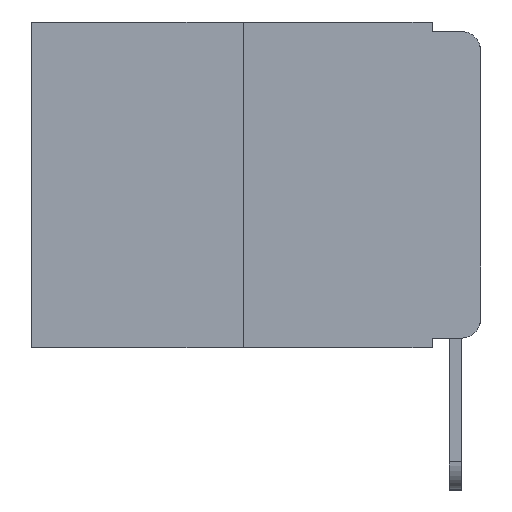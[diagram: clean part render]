
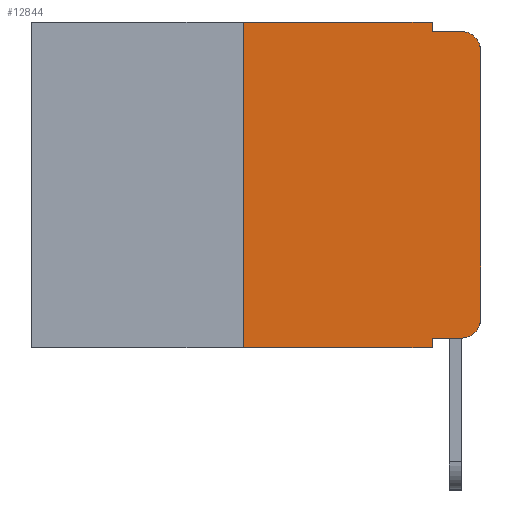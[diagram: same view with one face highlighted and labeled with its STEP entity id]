
A CAD part, left-side view. The second image highlights one B-rep face of the part: STEP entity #12844.
In plain terms, the highlighted planar face has unit normal (-1, 0, 0).
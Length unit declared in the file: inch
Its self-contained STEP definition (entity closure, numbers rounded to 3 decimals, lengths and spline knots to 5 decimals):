
#192 = EDGE_CURVE ( 'NONE', #21974, #3777, #5149, .T. ) ;
#531 = AXIS2_PLACEMENT_3D ( 'NONE', #17033, #23266, #1209 ) ;
#1209 = DIRECTION ( 'NONE',  ( 0., 0., -1. ) ) ;
#1304 = LINE ( 'NONE', #4498, #17083 ) ;
#1358 = DIRECTION ( 'NONE',  ( 0., -1., 0. ) ) ;
#1533 = ORIENTED_EDGE ( 'NONE', *, *, #21431, .T. ) ;
#1636 = CARTESIAN_POINT ( 'NONE',  ( 0., 0.051, -0.333 ) ) ;
#1869 = EDGE_CURVE ( 'NONE', #11235, #10809, #1304, .T. ) ;
#1993 = CARTESIAN_POINT ( 'NONE',  ( 0., 0.051, -0.343 ) ) ;
#3062 = CARTESIAN_POINT ( 'NONE',  ( 0., 0.051, 0. ) ) ;
#3777 = VERTEX_POINT ( 'NONE', #10928 ) ;
#4167 = LINE ( 'NONE', #24477, #11271 ) ;
#4286 = CARTESIAN_POINT ( 'NONE',  ( 0., 0., -0.313 ) ) ;
#4479 = VERTEX_POINT ( 'NONE', #4286 ) ;
#4498 = CARTESIAN_POINT ( 'NONE',  ( 0., 0.051, -0.01 ) ) ;
#4599 = ORIENTED_EDGE ( 'NONE', *, *, #22278, .T. ) ;
#4781 = EDGE_CURVE ( 'NONE', #16105, #11322, #20955, .T. ) ;
#5149 = LINE ( 'NONE', #25591, #25607 ) ;
#5235 = CARTESIAN_POINT ( 'NONE',  ( 0., 0.051, -0.333 ) ) ;
#5629 = VERTEX_POINT ( 'NONE', #13945 ) ;
#5670 = EDGE_CURVE ( 'NONE', #18080, #11235, #4167, .T. ) ;
#6289 = DIRECTION ( 'NONE',  ( 0., -1., 0. ) ) ;
#7380 = CARTESIAN_POINT ( 'NONE',  ( 0., 0.473, 0. ) ) ;
#7855 = CARTESIAN_POINT ( 'NONE',  ( 0., 0.051, -0.01 ) ) ;
#8781 = ORIENTED_EDGE ( 'NONE', *, *, #192, .F. ) ;
#9472 = AXIS2_PLACEMENT_3D ( 'NONE', #20008, #10299, #14383 ) ;
#9832 = DIRECTION ( 'NONE',  ( 0., 0., 1. ) ) ;
#10065 = CARTESIAN_POINT ( 'NONE',  ( 0., 0.02, -0.01 ) ) ;
#10299 = DIRECTION ( 'NONE',  ( -1., 0., 0. ) ) ;
#10809 = VERTEX_POINT ( 'NONE', #10065 ) ;
#10928 = CARTESIAN_POINT ( 'NONE',  ( 0., 0.25, 0. ) ) ;
#10940 = LINE ( 'NONE', #15917, #20232 ) ;
#10986 = DIRECTION ( 'NONE',  ( -1., 0., 0. ) ) ;
#11235 = VERTEX_POINT ( 'NONE', #7855 ) ;
#11271 = VECTOR ( 'NONE', #24227, 39.37008 ) ;
#11322 = VERTEX_POINT ( 'NONE', #1993 ) ;
#11356 = FACE_OUTER_BOUND ( 'NONE', #17373, .T. ) ;
#11830 = VERTEX_POINT ( 'NONE', #25258 ) ;
#12199 = DIRECTION ( 'NONE',  ( 0., -1., 0. ) ) ;
#12820 = DIRECTION ( 'NONE',  ( 0., 0., -1. ) ) ;
#12844 = ADVANCED_FACE ( 'NONE', ( #11356 ), #15232, .F. ) ;
#12852 = DIRECTION ( 'NONE',  ( 0., 0., -1. ) ) ;
#13000 = EDGE_CURVE ( 'NONE', #4479, #5629, #25000, .T. ) ;
#13093 = LINE ( 'NONE', #7380, #13714 ) ;
#13714 = VECTOR ( 'NONE', #23322, 39.37008 ) ;
#13728 = DIRECTION ( 'NONE',  ( 0., 0., 1. ) ) ;
#13945 = CARTESIAN_POINT ( 'NONE',  ( 0., 0., -0.03 ) ) ;
#14383 = DIRECTION ( 'NONE',  ( 0., 0., -1. ) ) ;
#15232 = PLANE ( 'NONE',  #531 ) ;
#15661 = CARTESIAN_POINT ( 'NONE',  ( 0., 0., 0. ) ) ;
#15702 = VECTOR ( 'NONE', #12852, 39.37008 ) ;
#15917 = CARTESIAN_POINT ( 'NONE',  ( 0., 0.473, -0.343 ) ) ;
#16000 = CARTESIAN_POINT ( 'NONE',  ( 0., 0.051, 0. ) ) ;
#16105 = VERTEX_POINT ( 'NONE', #1636 ) ;
#16619 = VECTOR ( 'NONE', #9832, 39.37008 ) ;
#16697 = CIRCLE ( 'NONE', #22462, 0.02 ) ;
#16748 = LINE ( 'NONE', #5235, #23246 ) ;
#17033 = CARTESIAN_POINT ( 'NONE',  ( 0., 0.473, 0. ) ) ;
#17083 = VECTOR ( 'NONE', #12199, 39.37008 ) ;
#17373 = EDGE_LOOP ( 'NONE', ( #22389, #18364, #23233, #20526, #22597, #8781, #20082, #24775, #4599, #1533 ) ) ;
#17891 = CARTESIAN_POINT ( 'NONE',  ( 0., 0.25, -0.343 ) ) ;
#18059 = EDGE_CURVE ( 'NONE', #21974, #11322, #10940, .T. ) ;
#18080 = VERTEX_POINT ( 'NONE', #16000 ) ;
#18364 = ORIENTED_EDGE ( 'NONE', *, *, #23373, .T. ) ;
#18526 = CIRCLE ( 'NONE', #9472, 0.02 ) ;
#19162 = EDGE_CURVE ( 'NONE', #3777, #18080, #13093, .T. ) ;
#20008 = CARTESIAN_POINT ( 'NONE',  ( 0., 0.02, -0.313 ) ) ;
#20082 = ORIENTED_EDGE ( 'NONE', *, *, #18059, .T. ) ;
#20232 = VECTOR ( 'NONE', #6289, 39.37008 ) ;
#20526 = ORIENTED_EDGE ( 'NONE', *, *, #5670, .F. ) ;
#20955 = LINE ( 'NONE', #3062, #15702 ) ;
#21431 = EDGE_CURVE ( 'NONE', #11830, #4479, #18526, .T. ) ;
#21974 = VERTEX_POINT ( 'NONE', #17891 ) ;
#22278 = EDGE_CURVE ( 'NONE', #16105, #11830, #16748, .T. ) ;
#22389 = ORIENTED_EDGE ( 'NONE', *, *, #13000, .T. ) ;
#22462 = AXIS2_PLACEMENT_3D ( 'NONE', #22942, #10986, #12820 ) ;
#22597 = ORIENTED_EDGE ( 'NONE', *, *, #19162, .F. ) ;
#22942 = CARTESIAN_POINT ( 'NONE',  ( 0., 0.02, -0.03 ) ) ;
#23233 = ORIENTED_EDGE ( 'NONE', *, *, #1869, .F. ) ;
#23246 = VECTOR ( 'NONE', #1358, 39.37008 ) ;
#23266 = DIRECTION ( 'NONE',  ( 1., 0., 0. ) ) ;
#23322 = DIRECTION ( 'NONE',  ( 0., -1., 0. ) ) ;
#23373 = EDGE_CURVE ( 'NONE', #5629, #10809, #16697, .T. ) ;
#24227 = DIRECTION ( 'NONE',  ( 0., 0., -1. ) ) ;
#24477 = CARTESIAN_POINT ( 'NONE',  ( 0., 0.051, 0. ) ) ;
#24775 = ORIENTED_EDGE ( 'NONE', *, *, #4781, .F. ) ;
#25000 = LINE ( 'NONE', #15661, #16619 ) ;
#25258 = CARTESIAN_POINT ( 'NONE',  ( 0., 0.02, -0.333 ) ) ;
#25591 = CARTESIAN_POINT ( 'NONE',  ( 0., 0.25, 0. ) ) ;
#25607 = VECTOR ( 'NONE', #13728, 39.37008 ) ;
